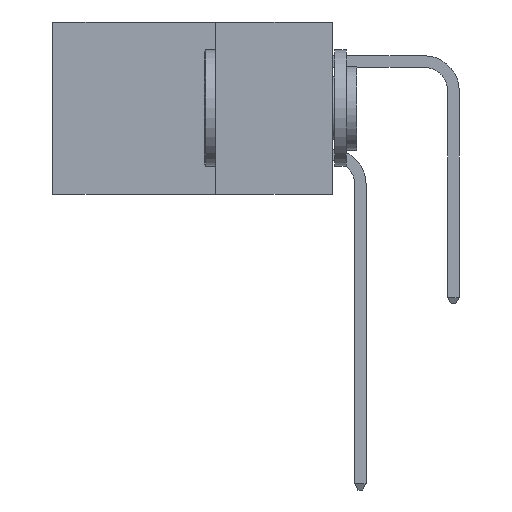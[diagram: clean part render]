
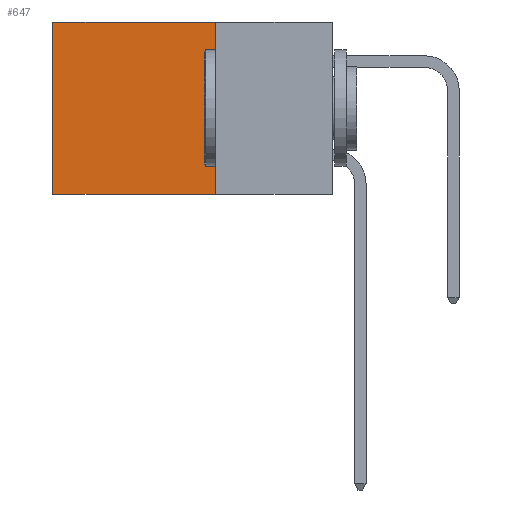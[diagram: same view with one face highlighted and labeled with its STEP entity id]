
A CAD part, left-side view. The second image highlights one B-rep face of the part: STEP entity #647.
In plain terms, the highlighted planar face has unit normal (-1, 0, 0).
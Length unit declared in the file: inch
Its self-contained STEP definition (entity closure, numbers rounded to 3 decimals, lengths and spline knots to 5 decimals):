
#61 = VERTEX_POINT ( 'NONE', #5822 ) ;
#162 = DIRECTION ( 'NONE',  ( 1., 0., 0. ) ) ;
#647 = ADVANCED_FACE ( 'NONE', ( #5332 ), #10208, .F. ) ;
#833 = VERTEX_POINT ( 'NONE', #4315 ) ;
#963 = EDGE_CURVE ( 'NONE', #61, #833, #10488, .T. ) ;
#1944 = CARTESIAN_POINT ( 'NONE',  ( 0.2615, 0.25, -0.37 ) ) ;
#2037 = VERTEX_POINT ( 'NONE', #12769 ) ;
#2528 = ORIENTED_EDGE ( 'NONE', *, *, #963, .T. ) ;
#2549 = LINE ( 'NONE', #7091, #11221 ) ;
#2875 = VECTOR ( 'NONE', #8848, 39.37008 ) ;
#3350 = AXIS2_PLACEMENT_3D ( 'NONE', #1944, #162, #13073 ) ;
#3644 = CARTESIAN_POINT ( 'NONE',  ( 0.2615, 0.6, -0.37 ) ) ;
#4315 = CARTESIAN_POINT ( 'NONE',  ( 0.2615, 0.6, 0. ) ) ;
#4443 = VECTOR ( 'NONE', #4564, 39.37008 ) ;
#4564 = DIRECTION ( 'NONE',  ( 0., 1., 0. ) ) ;
#5332 = FACE_OUTER_BOUND ( 'NONE', #11421, .T. ) ;
#5503 = LINE ( 'NONE', #8680, #2875 ) ;
#5516 = LINE ( 'NONE', #13215, #14052 ) ;
#5822 = CARTESIAN_POINT ( 'NONE',  ( 0.2615, 0.25, 0. ) ) ;
#7091 = CARTESIAN_POINT ( 'NONE',  ( 0.2615, 0.25, -0.37 ) ) ;
#7448 = DIRECTION ( 'NONE',  ( 0., 0., -1. ) ) ;
#7926 = EDGE_CURVE ( 'NONE', #61, #2037, #2549, .T. ) ;
#8680 = CARTESIAN_POINT ( 'NONE',  ( 0.2615, 0.25, -0.37 ) ) ;
#8848 = DIRECTION ( 'NONE',  ( 0., 1., 0. ) ) ;
#8921 = VERTEX_POINT ( 'NONE', #3644 ) ;
#9501 = ORIENTED_EDGE ( 'NONE', *, *, #7926, .F. ) ;
#9948 = EDGE_CURVE ( 'NONE', #833, #8921, #5516, .T. ) ;
#10208 = PLANE ( 'NONE',  #3350 ) ;
#10348 = EDGE_CURVE ( 'NONE', #2037, #8921, #5503, .T. ) ;
#10488 = LINE ( 'NONE', #13501, #4443 ) ;
#11221 = VECTOR ( 'NONE', #7448, 39.37008 ) ;
#11421 = EDGE_LOOP ( 'NONE', ( #13584, #13564, #9501, #2528 ) ) ;
#12769 = CARTESIAN_POINT ( 'NONE',  ( 0.2615, 0.25, -0.37 ) ) ;
#13073 = DIRECTION ( 'NONE',  ( 0., 0., -1. ) ) ;
#13147 = DIRECTION ( 'NONE',  ( 0., 0., -1. ) ) ;
#13215 = CARTESIAN_POINT ( 'NONE',  ( 0.2615, 0.6, -0.37 ) ) ;
#13501 = CARTESIAN_POINT ( 'NONE',  ( 0.2615, 0.25, 0. ) ) ;
#13564 = ORIENTED_EDGE ( 'NONE', *, *, #10348, .F. ) ;
#13584 = ORIENTED_EDGE ( 'NONE', *, *, #9948, .T. ) ;
#14052 = VECTOR ( 'NONE', #13147, 39.37008 ) ;
